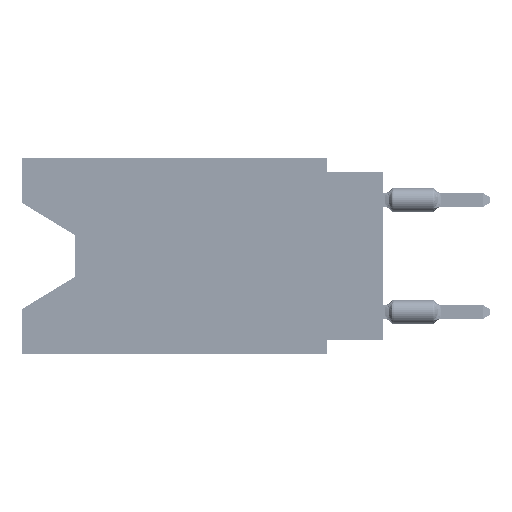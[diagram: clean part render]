
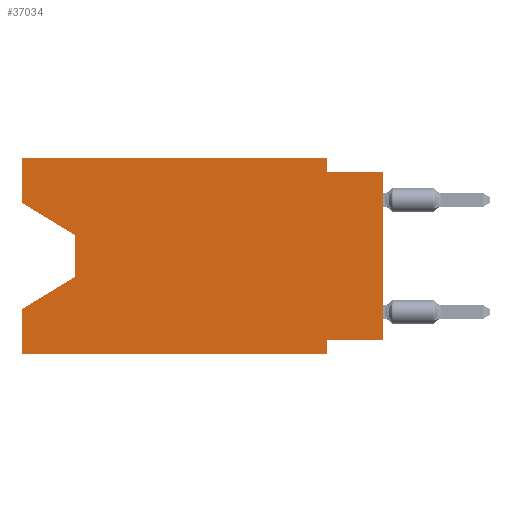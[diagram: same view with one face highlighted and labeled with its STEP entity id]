
A CAD part, left-side view. The second image highlights one B-rep face of the part: STEP entity #37034.
In plain terms, the highlighted planar face has unit normal (-1, 0, 0).
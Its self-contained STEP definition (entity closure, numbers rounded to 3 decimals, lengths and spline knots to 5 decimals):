
#1415 = LINE ( 'NONE', #99646, #6374 ) ;
#2395 = VERTEX_POINT ( 'NONE', #35209 ) ;
#3321 = DIRECTION ( 'NONE',  ( 0., 0., 1. ) ) ;
#3753 = CARTESIAN_POINT ( 'NONE',  ( 0., 0.645, 0. ) ) ;
#6374 = VECTOR ( 'NONE', #100202, 39.37008 ) ;
#8667 = DIRECTION ( 'NONE',  ( 0., 0., 1. ) ) ;
#9842 = CARTESIAN_POINT ( 'NONE',  ( 0., 0.645, -0.35 ) ) ;
#9849 = ORIENTED_EDGE ( 'NONE', *, *, #47843, .F. ) ;
#10644 = CARTESIAN_POINT ( 'NONE',  ( 0., 0.645, 0. ) ) ;
#10946 = DIRECTION ( 'NONE',  ( 0., -1., 0. ) ) ;
#11160 = LINE ( 'NONE', #45387, #61914 ) ;
#11508 = EDGE_LOOP ( 'NONE', ( #71009, #47500, #109645, #96814, #34942, #62558, #9849, #30864, #84022, #52851, #76181, #17990 ) ) ;
#11752 = VECTOR ( 'NONE', #77301, 39.37008 ) ;
#11770 = VERTEX_POINT ( 'NONE', #86726 ) ;
#11843 = VERTEX_POINT ( 'NONE', #99566 ) ;
#15030 = CARTESIAN_POINT ( 'NONE',  ( 0., 0.645, 0. ) ) ;
#15386 = EDGE_CURVE ( 'NONE', #30050, #69336, #68554, .T. ) ;
#17990 = ORIENTED_EDGE ( 'NONE', *, *, #47304, .F. ) ;
#21691 = FACE_OUTER_BOUND ( 'NONE', #11508, .T. ) ;
#22048 = EDGE_CURVE ( 'NONE', #11770, #30097, #88398, .T. ) ;
#24874 = CARTESIAN_POINT ( 'NONE',  ( 0., 0.1, -0.325 ) ) ;
#25353 = DIRECTION ( 'NONE',  ( 0., -1., 0. ) ) ;
#25916 = VECTOR ( 'NONE', #47033, 39.37008 ) ;
#27175 = LINE ( 'NONE', #42903, #105182 ) ;
#28605 = EDGE_CURVE ( 'NONE', #37448, #32849, #11160, .T. ) ;
#28858 = EDGE_CURVE ( 'NONE', #52875, #37448, #84597, .T. ) ;
#29877 = LINE ( 'NONE', #37181, #50915 ) ;
#30050 = VERTEX_POINT ( 'NONE', #58790 ) ;
#30097 = VERTEX_POINT ( 'NONE', #50931 ) ;
#30619 = EDGE_CURVE ( 'NONE', #11843, #30050, #1415, .T. ) ;
#30864 = ORIENTED_EDGE ( 'NONE', *, *, #44536, .T. ) ;
#31602 = VERTEX_POINT ( 'NONE', #106708 ) ;
#32849 = VERTEX_POINT ( 'NONE', #75223 ) ;
#33742 = DIRECTION ( 'NONE',  ( 0., 0., -1. ) ) ;
#33820 = CARTESIAN_POINT ( 'NONE',  ( 0., 0.645, 0. ) ) ;
#34170 = LINE ( 'NONE', #50456, #38191 ) ;
#34232 = VERTEX_POINT ( 'NONE', #108531 ) ;
#34942 = ORIENTED_EDGE ( 'NONE', *, *, #22048, .T. ) ;
#35209 = CARTESIAN_POINT ( 'NONE',  ( 0., 0., -0.325 ) ) ;
#37034 = ADVANCED_FACE ( 'NONE', ( #21691 ), #105382, .F. ) ;
#37181 = CARTESIAN_POINT ( 'NONE',  ( 0., 0., 0. ) ) ;
#37448 = VERTEX_POINT ( 'NONE', #97368 ) ;
#37649 = CARTESIAN_POINT ( 'NONE',  ( 0., 0., -0.325 ) ) ;
#38056 = DIRECTION ( 'NONE',  ( 0., 0., -1. ) ) ;
#38191 = VECTOR ( 'NONE', #41473, 39.37008 ) ;
#41473 = DIRECTION ( 'NONE',  ( 0., 0., -1. ) ) ;
#42903 = CARTESIAN_POINT ( 'NONE',  ( 0., 0.645, 0. ) ) ;
#44536 = EDGE_CURVE ( 'NONE', #2395, #34232, #29877, .T. ) ;
#45387 = CARTESIAN_POINT ( 'NONE',  ( 0., 0.1, 0. ) ) ;
#47033 = DIRECTION ( 'NONE',  ( 0., 0.855, -0.519 ) ) ;
#47304 = EDGE_CURVE ( 'NONE', #11843, #52875, #27175, .T. ) ;
#47500 = ORIENTED_EDGE ( 'NONE', *, *, #15386, .T. ) ;
#47843 = EDGE_CURVE ( 'NONE', #2395, #101739, #53974, .T. ) ;
#50456 = CARTESIAN_POINT ( 'NONE',  ( 0., 0.1, -0.35 ) ) ;
#50915 = VECTOR ( 'NONE', #88292, 39.37008 ) ;
#50931 = CARTESIAN_POINT ( 'NONE',  ( 0., 0.1, -0.35 ) ) ;
#52851 = ORIENTED_EDGE ( 'NONE', *, *, #28605, .F. ) ;
#52875 = VERTEX_POINT ( 'NONE', #33820 ) ;
#53974 = LINE ( 'NONE', #37649, #56841 ) ;
#56841 = VECTOR ( 'NONE', #64024, 39.37008 ) ;
#58790 = CARTESIAN_POINT ( 'NONE',  ( 0., 0.55, -0.138 ) ) ;
#61914 = VECTOR ( 'NONE', #38056, 39.37008 ) ;
#62558 = ORIENTED_EDGE ( 'NONE', *, *, #94885, .F. ) ;
#64024 = DIRECTION ( 'NONE',  ( 0., 1., 0. ) ) ;
#64351 = DIRECTION ( 'NONE',  ( 1., 0., 0. ) ) ;
#67881 = LINE ( 'NONE', #83603, #92177 ) ;
#68554 = LINE ( 'NONE', #102823, #97989 ) ;
#69336 = VERTEX_POINT ( 'NONE', #99647 ) ;
#70101 = VECTOR ( 'NONE', #10946, 39.37008 ) ;
#71009 = ORIENTED_EDGE ( 'NONE', *, *, #30619, .T. ) ;
#75223 = CARTESIAN_POINT ( 'NONE',  ( 0., 0.1, -0.025 ) ) ;
#76181 = ORIENTED_EDGE ( 'NONE', *, *, #28858, .F. ) ;
#77301 = DIRECTION ( 'NONE',  ( 0., -1., 0. ) ) ;
#80669 = DIRECTION ( 'NONE',  ( 0., 0., -1. ) ) ;
#83603 = CARTESIAN_POINT ( 'NONE',  ( 0., 0., -0.025 ) ) ;
#83665 = EDGE_CURVE ( 'NONE', #32849, #34232, #67881, .T. ) ;
#83920 = EDGE_CURVE ( 'NONE', #69336, #31602, #104364, .T. ) ;
#84022 = ORIENTED_EDGE ( 'NONE', *, *, #83665, .F. ) ;
#84597 = LINE ( 'NONE', #15030, #11752 ) ;
#86726 = CARTESIAN_POINT ( 'NONE',  ( 0., 0.645, -0.35 ) ) ;
#88292 = DIRECTION ( 'NONE',  ( 0., 0., 1. ) ) ;
#88398 = LINE ( 'NONE', #9842, #70101 ) ;
#89971 = VECTOR ( 'NONE', #3321, 39.37008 ) ;
#92177 = VECTOR ( 'NONE', #25353, 39.37008 ) ;
#93523 = EDGE_CURVE ( 'NONE', #11770, #31602, #97056, .T. ) ;
#94885 = EDGE_CURVE ( 'NONE', #101739, #30097, #34170, .T. ) ;
#95930 = CARTESIAN_POINT ( 'NONE',  ( 0., 0.55, -0.212 ) ) ;
#96814 = ORIENTED_EDGE ( 'NONE', *, *, #93523, .F. ) ;
#97056 = LINE ( 'NONE', #10644, #89971 ) ;
#97368 = CARTESIAN_POINT ( 'NONE',  ( 0., 0.1, 0. ) ) ;
#97989 = VECTOR ( 'NONE', #33742, 39.37008 ) ;
#99566 = CARTESIAN_POINT ( 'NONE',  ( 0., 0.645, -0.08025 ) ) ;
#99646 = CARTESIAN_POINT ( 'NONE',  ( 0., 0.645, -0.08025 ) ) ;
#99647 = CARTESIAN_POINT ( 'NONE',  ( 0., 0.55, -0.212 ) ) ;
#100202 = DIRECTION ( 'NONE',  ( 0., -0.855, -0.519 ) ) ;
#100338 = AXIS2_PLACEMENT_3D ( 'NONE', #3753, #64351, #80669 ) ;
#101739 = VERTEX_POINT ( 'NONE', #24874 ) ;
#102823 = CARTESIAN_POINT ( 'NONE',  ( 0., 0.55, -0.138 ) ) ;
#104364 = LINE ( 'NONE', #95930, #25916 ) ;
#105182 = VECTOR ( 'NONE', #8667, 39.37008 ) ;
#105382 = PLANE ( 'NONE',  #100338 ) ;
#106708 = CARTESIAN_POINT ( 'NONE',  ( 0., 0.645, -0.26975 ) ) ;
#108531 = CARTESIAN_POINT ( 'NONE',  ( 0., 0., -0.025 ) ) ;
#109645 = ORIENTED_EDGE ( 'NONE', *, *, #83920, .T. ) ;
